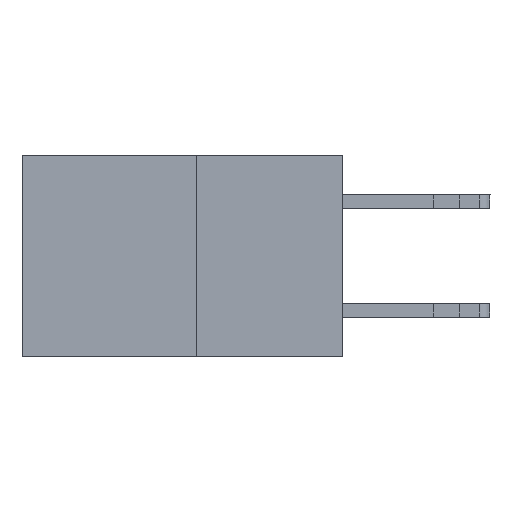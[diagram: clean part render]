
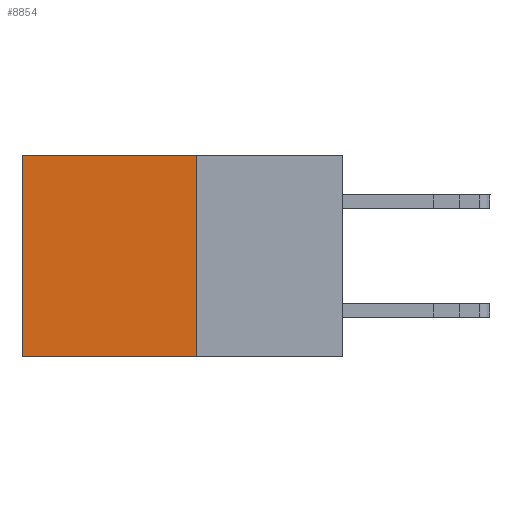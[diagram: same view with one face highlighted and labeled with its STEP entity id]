
A CAD part, left-side view. The second image highlights one B-rep face of the part: STEP entity #8854.
In plain terms, the highlighted planar face has unit normal (-1, 0, 0).
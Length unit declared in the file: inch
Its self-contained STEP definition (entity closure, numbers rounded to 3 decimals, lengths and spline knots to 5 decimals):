
#370 = VECTOR ( 'NONE', #4197, 39.37008 ) ;
#1560 = FACE_OUTER_BOUND ( 'NONE', #1858, .T. ) ;
#1858 = EDGE_LOOP ( 'NONE', ( #3806, #6139, #8070, #14429 ) ) ;
#2007 = VERTEX_POINT ( 'NONE', #7645 ) ;
#3806 = ORIENTED_EDGE ( 'NONE', *, *, #4067, .T. ) ;
#4067 = EDGE_CURVE ( 'NONE', #6922, #10839, #10773, .T. ) ;
#4197 = DIRECTION ( 'NONE',  ( 0., 1., 0. ) ) ;
#4390 = DIRECTION ( 'NONE',  ( 0., 0., -1. ) ) ;
#4405 = EDGE_CURVE ( 'NONE', #5471, #2007, #12466, .T. ) ;
#4503 = CARTESIAN_POINT ( 'NONE',  ( 0.277, 0.27, -0.37 ) ) ;
#5051 = LINE ( 'NONE', #16265, #8886 ) ;
#5471 = VERTEX_POINT ( 'NONE', #6569 ) ;
#6139 = ORIENTED_EDGE ( 'NONE', *, *, #13060, .F. ) ;
#6569 = CARTESIAN_POINT ( 'NONE',  ( 0.277, 0.27, 0. ) ) ;
#6783 = PLANE ( 'NONE',  #8433 ) ;
#6922 = VERTEX_POINT ( 'NONE', #10275 ) ;
#7098 = DIRECTION ( 'NONE',  ( 0., 0., -1. ) ) ;
#7645 = CARTESIAN_POINT ( 'NONE',  ( 0.277, 0.27, -0.37 ) ) ;
#8070 = ORIENTED_EDGE ( 'NONE', *, *, #4405, .F. ) ;
#8121 = DIRECTION ( 'NONE',  ( 0., 0., -1. ) ) ;
#8234 = LINE ( 'NONE', #14741, #370 ) ;
#8433 = AXIS2_PLACEMENT_3D ( 'NONE', #4503, #9368, #8121 ) ;
#8854 = ADVANCED_FACE ( 'NONE', ( #1560 ), #6783, .F. ) ;
#8886 = VECTOR ( 'NONE', #12609, 39.37008 ) ;
#9096 = VECTOR ( 'NONE', #7098, 39.37008 ) ;
#9124 = CARTESIAN_POINT ( 'NONE',  ( 0.277, 0.59, -0.37 ) ) ;
#9368 = DIRECTION ( 'NONE',  ( 1., 0., 0. ) ) ;
#10275 = CARTESIAN_POINT ( 'NONE',  ( 0.277, 0.59, 0. ) ) ;
#10773 = LINE ( 'NONE', #15857, #14242 ) ;
#10839 = VERTEX_POINT ( 'NONE', #9124 ) ;
#11200 = CARTESIAN_POINT ( 'NONE',  ( 0.277, 0.27, -0.37 ) ) ;
#12466 = LINE ( 'NONE', #11200, #9096 ) ;
#12609 = DIRECTION ( 'NONE',  ( 0., 1., 0. ) ) ;
#13060 = EDGE_CURVE ( 'NONE', #2007, #10839, #8234, .T. ) ;
#14242 = VECTOR ( 'NONE', #4390, 39.37008 ) ;
#14429 = ORIENTED_EDGE ( 'NONE', *, *, #14455, .T. ) ;
#14455 = EDGE_CURVE ( 'NONE', #5471, #6922, #5051, .T. ) ;
#14741 = CARTESIAN_POINT ( 'NONE',  ( 0.277, 0.27, -0.37 ) ) ;
#15857 = CARTESIAN_POINT ( 'NONE',  ( 0.277, 0.59, -0.37 ) ) ;
#16265 = CARTESIAN_POINT ( 'NONE',  ( 0.277, 0.27, 0. ) ) ;
